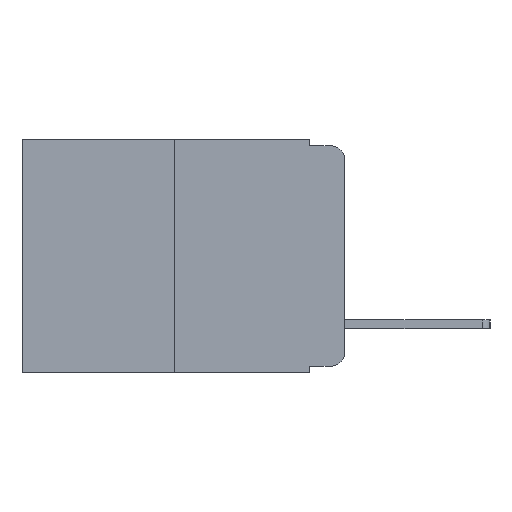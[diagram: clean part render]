
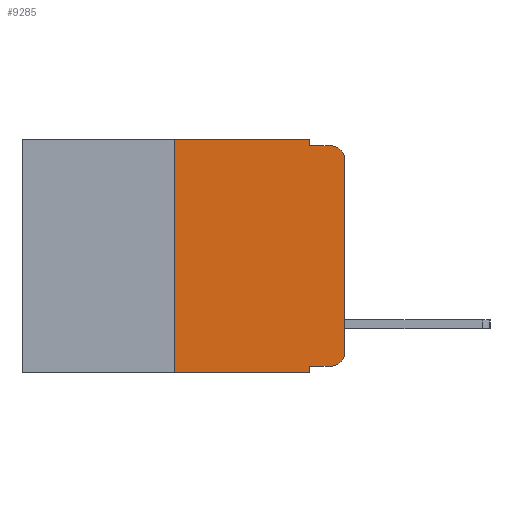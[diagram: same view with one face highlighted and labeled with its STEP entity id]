
A CAD part, left-side view. The second image highlights one B-rep face of the part: STEP entity #9285.
In plain terms, the highlighted planar face has unit normal (-1, 0, 0).
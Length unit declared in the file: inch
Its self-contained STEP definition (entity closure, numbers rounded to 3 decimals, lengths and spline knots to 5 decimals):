
#88 = EDGE_CURVE ( 'NONE', #758, #16406, #8347, .T. ) ;
#98 = VECTOR ( 'NONE', #10344, 39.37008 ) ;
#269 = CARTESIAN_POINT ( 'NONE',  ( 0., 0.051, 0. ) ) ;
#485 = VERTEX_POINT ( 'NONE', #5254 ) ;
#758 = VERTEX_POINT ( 'NONE', #17899 ) ;
#943 = CARTESIAN_POINT ( 'NONE',  ( 0., 0.473, -0.343 ) ) ;
#1127 = CARTESIAN_POINT ( 'NONE',  ( 0., 0.25, 0. ) ) ;
#1489 = EDGE_CURVE ( 'NONE', #16406, #18334, #4335, .T. ) ;
#1515 = AXIS2_PLACEMENT_3D ( 'NONE', #11187, #1691, #12622 ) ;
#1635 = PLANE ( 'NONE',  #3845 ) ;
#1691 = DIRECTION ( 'NONE',  ( -1., 0., 0. ) ) ;
#1791 = CIRCLE ( 'NONE', #9302, 0.02 ) ;
#2047 = CARTESIAN_POINT ( 'NONE',  ( 0., 0.02, -0.333 ) ) ;
#2131 = CARTESIAN_POINT ( 'NONE',  ( 0., 0., -0.313 ) ) ;
#2940 = LINE ( 'NONE', #269, #17950 ) ;
#3004 = VECTOR ( 'NONE', #10850, 39.37008 ) ;
#3292 = DIRECTION ( 'NONE',  ( 0., 0., 1. ) ) ;
#3815 = VERTEX_POINT ( 'NONE', #2131 ) ;
#3844 = CARTESIAN_POINT ( 'NONE',  ( 0., 0.473, 0. ) ) ;
#3845 = AXIS2_PLACEMENT_3D ( 'NONE', #14000, #16836, #8223 ) ;
#3874 = LINE ( 'NONE', #11091, #6711 ) ;
#3938 = DIRECTION ( 'NONE',  ( 0., -1., 0. ) ) ;
#4147 = CARTESIAN_POINT ( 'NONE',  ( 0., 0., -0.03 ) ) ;
#4335 = LINE ( 'NONE', #3844, #12896 ) ;
#4388 = ORIENTED_EDGE ( 'NONE', *, *, #6905, .F. ) ;
#4717 = VECTOR ( 'NONE', #13859, 39.37008 ) ;
#4732 = EDGE_CURVE ( 'NONE', #15462, #18970, #9311, .T. ) ;
#5254 = CARTESIAN_POINT ( 'NONE',  ( 0., 0.051, -0.343 ) ) ;
#5362 = DIRECTION ( 'NONE',  ( 0., 0., -1. ) ) ;
#5497 = VERTEX_POINT ( 'NONE', #2047 ) ;
#5680 = CARTESIAN_POINT ( 'NONE',  ( 0., 0.051, 0. ) ) ;
#5754 = EDGE_CURVE ( 'NONE', #14266, #5497, #11343, .T. ) ;
#5847 = CARTESIAN_POINT ( 'NONE',  ( 0., 0.25, 0. ) ) ;
#6033 = DIRECTION ( 'NONE',  ( 0., -1., 0. ) ) ;
#6277 = CARTESIAN_POINT ( 'NONE',  ( 0., 0.051, -0.333 ) ) ;
#6711 = VECTOR ( 'NONE', #3292, 39.37008 ) ;
#6905 = EDGE_CURVE ( 'NONE', #14266, #485, #2940, .T. ) ;
#7073 = ORIENTED_EDGE ( 'NONE', *, *, #88, .F. ) ;
#7623 = EDGE_CURVE ( 'NONE', #758, #485, #15458, .T. ) ;
#7920 = CIRCLE ( 'NONE', #1515, 0.02 ) ;
#8016 = CARTESIAN_POINT ( 'NONE',  ( 0., 0.051, 0. ) ) ;
#8223 = DIRECTION ( 'NONE',  ( 0., 0., -1. ) ) ;
#8272 = ORIENTED_EDGE ( 'NONE', *, *, #10936, .F. ) ;
#8347 = LINE ( 'NONE', #5847, #98 ) ;
#9285 = ADVANCED_FACE ( 'NONE', ( #12758 ), #1635, .F. ) ;
#9302 = AXIS2_PLACEMENT_3D ( 'NONE', #9432, #19434, #10941 ) ;
#9311 = LINE ( 'NONE', #18837, #16023 ) ;
#9348 = LINE ( 'NONE', #8016, #4717 ) ;
#9432 = CARTESIAN_POINT ( 'NONE',  ( 0., 0.02, -0.03 ) ) ;
#9751 = ORIENTED_EDGE ( 'NONE', *, *, #10870, .T. ) ;
#10344 = DIRECTION ( 'NONE',  ( 0., 0., 1. ) ) ;
#10850 = DIRECTION ( 'NONE',  ( 0., -1., 0. ) ) ;
#10870 = EDGE_CURVE ( 'NONE', #13062, #18970, #1791, .T. ) ;
#10936 = EDGE_CURVE ( 'NONE', #18334, #15462, #9348, .T. ) ;
#10941 = DIRECTION ( 'NONE',  ( 0., 0., -1. ) ) ;
#11055 = ORIENTED_EDGE ( 'NONE', *, *, #7623, .T. ) ;
#11091 = CARTESIAN_POINT ( 'NONE',  ( 0., 0., 0. ) ) ;
#11187 = CARTESIAN_POINT ( 'NONE',  ( 0., 0.02, -0.313 ) ) ;
#11343 = LINE ( 'NONE', #6277, #3004 ) ;
#11459 = ORIENTED_EDGE ( 'NONE', *, *, #1489, .F. ) ;
#11685 = VECTOR ( 'NONE', #6033, 39.37008 ) ;
#11824 = EDGE_CURVE ( 'NONE', #3815, #13062, #3874, .T. ) ;
#12622 = DIRECTION ( 'NONE',  ( 0., 0., -1. ) ) ;
#12758 = FACE_OUTER_BOUND ( 'NONE', #18302, .T. ) ;
#12896 = VECTOR ( 'NONE', #3938, 39.37008 ) ;
#13062 = VERTEX_POINT ( 'NONE', #4147 ) ;
#13304 = DIRECTION ( 'NONE',  ( 0., -1., 0. ) ) ;
#13859 = DIRECTION ( 'NONE',  ( 0., 0., -1. ) ) ;
#14000 = CARTESIAN_POINT ( 'NONE',  ( 0., 0.473, 0. ) ) ;
#14161 = ORIENTED_EDGE ( 'NONE', *, *, #11824, .T. ) ;
#14266 = VERTEX_POINT ( 'NONE', #19263 ) ;
#15025 = ORIENTED_EDGE ( 'NONE', *, *, #18823, .T. ) ;
#15458 = LINE ( 'NONE', #943, #11685 ) ;
#15462 = VERTEX_POINT ( 'NONE', #17491 ) ;
#16023 = VECTOR ( 'NONE', #13304, 39.37008 ) ;
#16282 = ORIENTED_EDGE ( 'NONE', *, *, #4732, .F. ) ;
#16406 = VERTEX_POINT ( 'NONE', #1127 ) ;
#16836 = DIRECTION ( 'NONE',  ( 1., 0., 0. ) ) ;
#17491 = CARTESIAN_POINT ( 'NONE',  ( 0., 0.051, -0.01 ) ) ;
#17853 = ORIENTED_EDGE ( 'NONE', *, *, #5754, .T. ) ;
#17899 = CARTESIAN_POINT ( 'NONE',  ( 0., 0.25, -0.343 ) ) ;
#17950 = VECTOR ( 'NONE', #5362, 39.37008 ) ;
#18302 = EDGE_LOOP ( 'NONE', ( #14161, #9751, #16282, #8272, #11459, #7073, #11055, #4388, #17853, #15025 ) ) ;
#18334 = VERTEX_POINT ( 'NONE', #5680 ) ;
#18556 = CARTESIAN_POINT ( 'NONE',  ( 0., 0.02, -0.01 ) ) ;
#18823 = EDGE_CURVE ( 'NONE', #5497, #3815, #7920, .T. ) ;
#18837 = CARTESIAN_POINT ( 'NONE',  ( 0., 0.051, -0.01 ) ) ;
#18970 = VERTEX_POINT ( 'NONE', #18556 ) ;
#19263 = CARTESIAN_POINT ( 'NONE',  ( 0., 0.051, -0.333 ) ) ;
#19434 = DIRECTION ( 'NONE',  ( -1., 0., 0. ) ) ;
